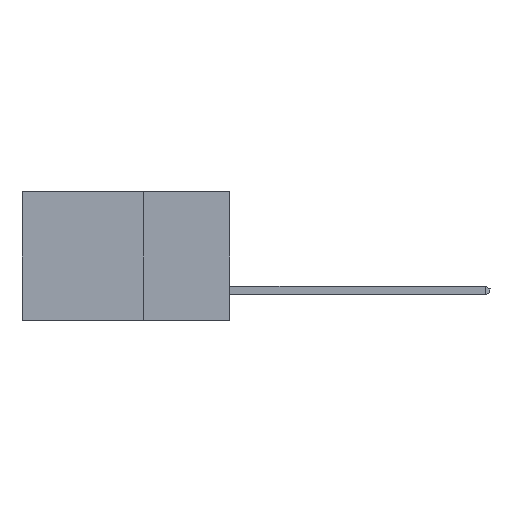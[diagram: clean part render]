
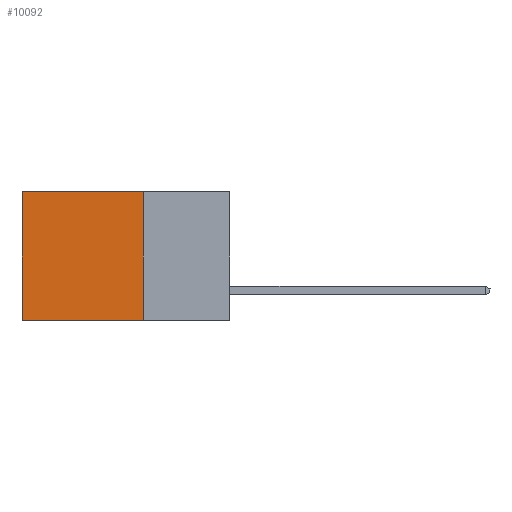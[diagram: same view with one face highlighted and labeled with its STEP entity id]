
A CAD part, left-side view. The second image highlights one B-rep face of the part: STEP entity #10092.
In plain terms, the highlighted planar face has unit normal (-1, 0, 0).
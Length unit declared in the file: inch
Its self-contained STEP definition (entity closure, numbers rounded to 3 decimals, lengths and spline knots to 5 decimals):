
#856 = CARTESIAN_POINT ( 'NONE',  ( 0.2615, 0.25, -0.37 ) ) ;
#1296 = DIRECTION ( 'NONE',  ( 0., 1., 0. ) ) ;
#1612 = VERTEX_POINT ( 'NONE', #18454 ) ;
#1885 = ORIENTED_EDGE ( 'NONE', *, *, #10774, .T. ) ;
#1959 = ORIENTED_EDGE ( 'NONE', *, *, #10485, .T. ) ;
#2296 = LINE ( 'NONE', #856, #12712 ) ;
#2795 = LINE ( 'NONE', #15064, #9150 ) ;
#3542 = DIRECTION ( 'NONE',  ( 0., 0., -1. ) ) ;
#3760 = DIRECTION ( 'NONE',  ( 0., 1., 0. ) ) ;
#3825 = ORIENTED_EDGE ( 'NONE', *, *, #7976, .F. ) ;
#3830 = VERTEX_POINT ( 'NONE', #19945 ) ;
#4015 = VERTEX_POINT ( 'NONE', #16142 ) ;
#4042 = DIRECTION ( 'NONE',  ( 0., 0., -1. ) ) ;
#4842 = LINE ( 'NONE', #9374, #7170 ) ;
#5262 = CARTESIAN_POINT ( 'NONE',  ( 0.2615, 0.25, -0.37 ) ) ;
#6121 = CARTESIAN_POINT ( 'NONE',  ( 0.2615, 0.25, 0. ) ) ;
#6382 = ORIENTED_EDGE ( 'NONE', *, *, #10364, .F. ) ;
#7170 = VECTOR ( 'NONE', #15477, 39.37008 ) ;
#7976 = EDGE_CURVE ( 'NONE', #1612, #15592, #2296, .T. ) ;
#8459 = DIRECTION ( 'NONE',  ( 1., 0., 0. ) ) ;
#9150 = VECTOR ( 'NONE', #4042, 39.37008 ) ;
#9374 = CARTESIAN_POINT ( 'NONE',  ( 0.2615, 0.6, -0.37 ) ) ;
#10092 = ADVANCED_FACE ( 'NONE', ( #19066 ), #16000, .F. ) ;
#10131 = VECTOR ( 'NONE', #1296, 39.37008 ) ;
#10364 = EDGE_CURVE ( 'NONE', #3830, #1612, #2795, .T. ) ;
#10485 = EDGE_CURVE ( 'NONE', #4015, #15592, #4842, .T. ) ;
#10774 = EDGE_CURVE ( 'NONE', #3830, #4015, #15322, .T. ) ;
#12712 = VECTOR ( 'NONE', #3760, 39.37008 ) ;
#15064 = CARTESIAN_POINT ( 'NONE',  ( 0.2615, 0.25, -0.37 ) ) ;
#15322 = LINE ( 'NONE', #6121, #10131 ) ;
#15477 = DIRECTION ( 'NONE',  ( 0., 0., -1. ) ) ;
#15592 = VERTEX_POINT ( 'NONE', #19621 ) ;
#15650 = AXIS2_PLACEMENT_3D ( 'NONE', #5262, #8459, #3542 ) ;
#16000 = PLANE ( 'NONE',  #15650 ) ;
#16142 = CARTESIAN_POINT ( 'NONE',  ( 0.2615, 0.6, 0. ) ) ;
#16743 = EDGE_LOOP ( 'NONE', ( #1959, #3825, #6382, #1885 ) ) ;
#18454 = CARTESIAN_POINT ( 'NONE',  ( 0.2615, 0.25, -0.37 ) ) ;
#19066 = FACE_OUTER_BOUND ( 'NONE', #16743, .T. ) ;
#19621 = CARTESIAN_POINT ( 'NONE',  ( 0.2615, 0.6, -0.37 ) ) ;
#19945 = CARTESIAN_POINT ( 'NONE',  ( 0.2615, 0.25, 0. ) ) ;
